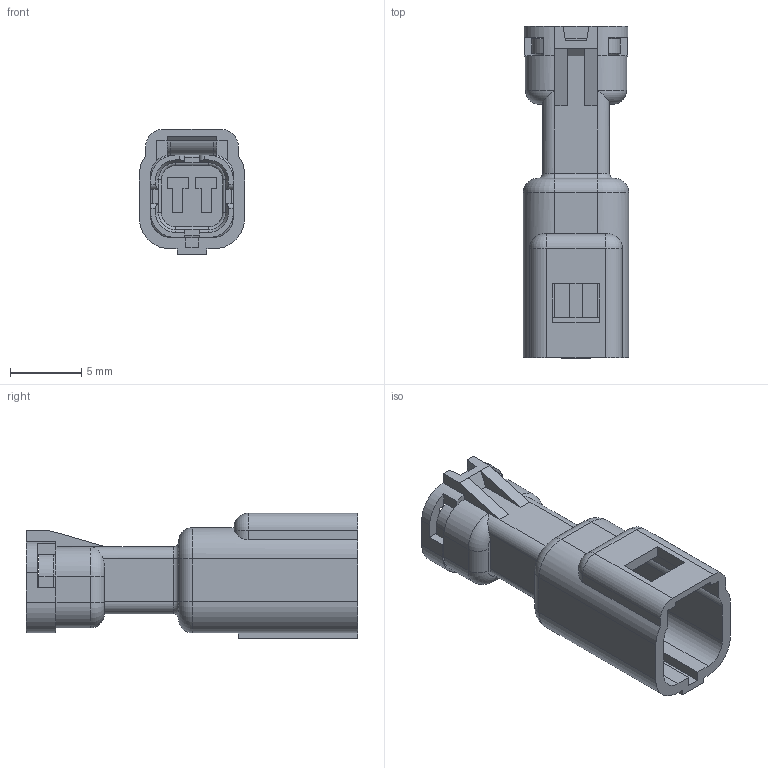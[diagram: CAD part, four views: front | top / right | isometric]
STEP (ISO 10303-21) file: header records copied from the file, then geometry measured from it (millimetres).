
FILE_DESCRIPTION (( 'STEP AP203' ), '1' );
FILE_NAME ('566-002-000-710.STEP', '2021-09-21T15:37:03', ( '' ), ( '' ), 'SwSTEP 2.0', 'SolidWorks 2020', '' );
FILE_SCHEMA (( 'CONFIG_CONTROL_DESIGN' ));
Length unit declared in the file: millimetre
Products named in the file (1): 566-002-000-710
Bounding box: 7.4 x 23.3 x 8.8 mm (x, y, z)
Volume: 612.6 mm3; surface area: 1512.3 mm2
Topology: 3 solids, 3 shells, 602 faces, 1472 edges, 874 vertices
Faces by surface type: plane 309, cylinder 173, torus 98, cone 20, bspline 2
Entity records: 17707 total; most frequent: CARTESIAN_POINT 3393, DIRECTION 3042, ORIENTED_EDGE 2944, EDGE_CURVE 1472, AXIS2_PLACEMENT_3D 1041, VECTOR 960, LINE 960, VERTEX_POINT 874
